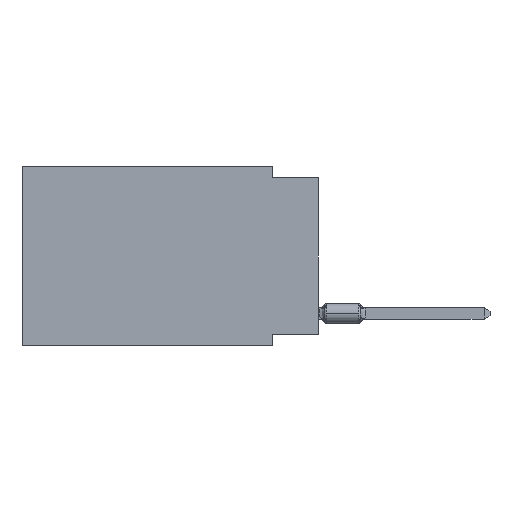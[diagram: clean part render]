
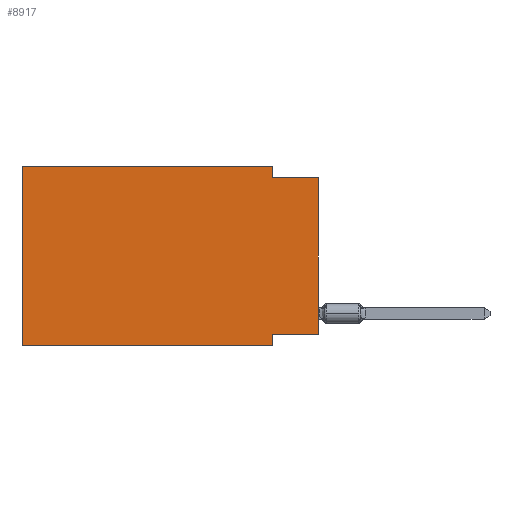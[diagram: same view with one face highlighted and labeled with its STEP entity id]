
A CAD part, left-side view. The second image highlights one B-rep face of the part: STEP entity #8917.
In plain terms, the highlighted planar face has unit normal (-1, 0, 0).
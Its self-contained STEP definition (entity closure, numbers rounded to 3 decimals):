
#81 = VERTEX_POINT ( 'NONE', #18746 ) ;
#654 = ORIENTED_EDGE ( 'NONE', *, *, #23425, .F. ) ;
#919 = VERTEX_POINT ( 'NONE', #5693 ) ;
#1195 = ORIENTED_EDGE ( 'NONE', *, *, #7394, .F. ) ;
#1206 = PLANE ( 'NONE',  #1688 ) ;
#1688 = AXIS2_PLACEMENT_3D ( 'NONE', #3364, #23179, #6485 ) ;
#2765 = CARTESIAN_POINT ( 'NONE',  ( 0., 2.54, -0.635 ) ) ;
#2891 = LINE ( 'NONE', #19692, #17153 ) ;
#3364 = CARTESIAN_POINT ( 'NONE',  ( 0., 16.383, 0. ) ) ;
#3780 = DIRECTION ( 'NONE',  ( 0., 1., 0. ) ) ;
#4069 = DIRECTION ( 'NONE',  ( 0., -1., 0. ) ) ;
#4158 = VERTEX_POINT ( 'NONE', #4732 ) ;
#4182 = CARTESIAN_POINT ( 'NONE',  ( 0., 16.383, -9.906 ) ) ;
#4185 = DIRECTION ( 'NONE',  ( 0., 0., 1. ) ) ;
#4732 = CARTESIAN_POINT ( 'NONE',  ( 0., 2.54, -9.271 ) ) ;
#5348 = ORIENTED_EDGE ( 'NONE', *, *, #13642, .F. ) ;
#5566 = CARTESIAN_POINT ( 'NONE',  ( 0., 0., -9.271 ) ) ;
#5612 = DIRECTION ( 'NONE',  ( 0., 0., -1. ) ) ;
#5693 = CARTESIAN_POINT ( 'NONE',  ( 0., 0., -0.635 ) ) ;
#6186 = VECTOR ( 'NONE', #3780, 1000. ) ;
#6485 = DIRECTION ( 'NONE',  ( 0., 0., -1. ) ) ;
#6518 = EDGE_CURVE ( 'NONE', #19046, #15434, #22573, .T. ) ;
#6720 = DIRECTION ( 'NONE',  ( 0., -1., 0. ) ) ;
#7119 = CARTESIAN_POINT ( 'NONE',  ( 0., 2.54, 0. ) ) ;
#7394 = EDGE_CURVE ( 'NONE', #20131, #4158, #20243, .T. ) ;
#7542 = CARTESIAN_POINT ( 'NONE',  ( 0., 16.383, 0. ) ) ;
#7653 = LINE ( 'NONE', #4182, #22038 ) ;
#7727 = DIRECTION ( 'NONE',  ( 0., 0., -1. ) ) ;
#8917 = ADVANCED_FACE ( 'NONE', ( #19353 ), #1206, .F. ) ;
#9169 = EDGE_CURVE ( 'NONE', #19046, #81, #7653, .T. ) ;
#9773 = EDGE_CURVE ( 'NONE', #19771, #11762, #16688, .T. ) ;
#9823 = ORIENTED_EDGE ( 'NONE', *, *, #9169, .T. ) ;
#9870 = ORIENTED_EDGE ( 'NONE', *, *, #23078, .T. ) ;
#10033 = VECTOR ( 'NONE', #21292, 1000. ) ;
#11149 = CARTESIAN_POINT ( 'NONE',  ( 0., 16.383, -9.906 ) ) ;
#11394 = CARTESIAN_POINT ( 'NONE',  ( 0., 16.383, 0. ) ) ;
#11762 = VERTEX_POINT ( 'NONE', #2765 ) ;
#12994 = DIRECTION ( 'NONE',  ( 0., -1., 0. ) ) ;
#13642 = EDGE_CURVE ( 'NONE', #11762, #919, #20075, .T. ) ;
#13964 = CARTESIAN_POINT ( 'NONE',  ( 0., 0., 0. ) ) ;
#14599 = LINE ( 'NONE', #18326, #18185 ) ;
#14879 = CARTESIAN_POINT ( 'NONE',  ( 0., 2.54, 0. ) ) ;
#15434 = VERTEX_POINT ( 'NONE', #11394 ) ;
#16082 = ORIENTED_EDGE ( 'NONE', *, *, #21081, .F. ) ;
#16688 = LINE ( 'NONE', #14879, #20534 ) ;
#17153 = VECTOR ( 'NONE', #6720, 1000. ) ;
#17651 = CARTESIAN_POINT ( 'NONE',  ( 0., 0., -9.271 ) ) ;
#18185 = VECTOR ( 'NONE', #7727, 1000. ) ;
#18326 = CARTESIAN_POINT ( 'NONE',  ( 0., 2.54, -9.906 ) ) ;
#18372 = ORIENTED_EDGE ( 'NONE', *, *, #6518, .F. ) ;
#18384 = ORIENTED_EDGE ( 'NONE', *, *, #9773, .F. ) ;
#18658 = VECTOR ( 'NONE', #4185, 1000. ) ;
#18746 = CARTESIAN_POINT ( 'NONE',  ( 0., 2.54, -9.906 ) ) ;
#19020 = VECTOR ( 'NONE', #12994, 1000. ) ;
#19046 = VERTEX_POINT ( 'NONE', #11149 ) ;
#19353 = FACE_OUTER_BOUND ( 'NONE', #21703, .T. ) ;
#19692 = CARTESIAN_POINT ( 'NONE',  ( 0., 16.383, 0. ) ) ;
#19771 = VERTEX_POINT ( 'NONE', #7119 ) ;
#20075 = LINE ( 'NONE', #22336, #19020 ) ;
#20131 = VERTEX_POINT ( 'NONE', #17651 ) ;
#20243 = LINE ( 'NONE', #5566, #6186 ) ;
#20534 = VECTOR ( 'NONE', #5612, 1000. ) ;
#21081 = EDGE_CURVE ( 'NONE', #4158, #81, #14599, .T. ) ;
#21292 = DIRECTION ( 'NONE',  ( 0., 0., 1. ) ) ;
#21703 = EDGE_LOOP ( 'NONE', ( #9870, #5348, #18384, #654, #18372, #9823, #16082, #1195 ) ) ;
#22038 = VECTOR ( 'NONE', #4069, 1000. ) ;
#22336 = CARTESIAN_POINT ( 'NONE',  ( 0., 0., -0.635 ) ) ;
#22573 = LINE ( 'NONE', #7542, #18658 ) ;
#23078 = EDGE_CURVE ( 'NONE', #20131, #919, #23079, .T. ) ;
#23079 = LINE ( 'NONE', #13964, #10033 ) ;
#23179 = DIRECTION ( 'NONE',  ( 1., 0., 0. ) ) ;
#23425 = EDGE_CURVE ( 'NONE', #15434, #19771, #2891, .T. ) ;
